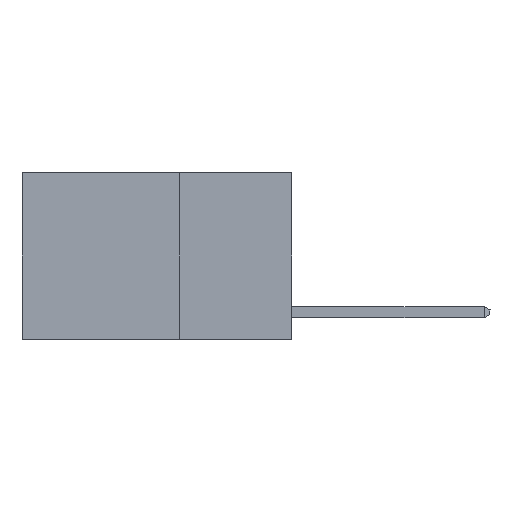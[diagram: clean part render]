
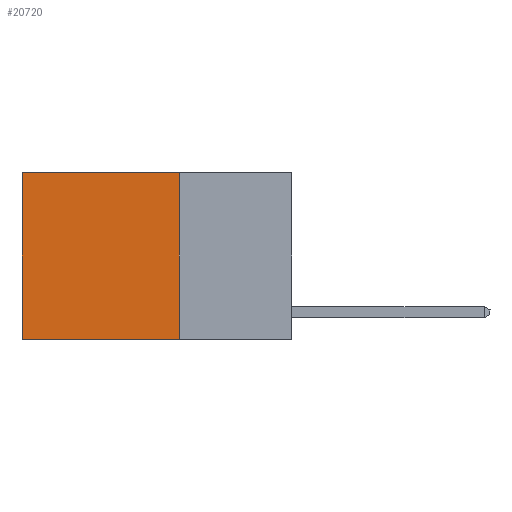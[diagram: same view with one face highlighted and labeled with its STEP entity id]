
A CAD part, left-side view. The second image highlights one B-rep face of the part: STEP entity #20720.
In plain terms, the highlighted planar face has unit normal (-1, 0, 0).
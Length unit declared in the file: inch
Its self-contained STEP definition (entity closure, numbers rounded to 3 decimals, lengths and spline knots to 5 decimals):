
#1170 = DIRECTION ( 'NONE',  ( 0., 0., -1. ) ) ;
#1508 = EDGE_CURVE ( 'NONE', #13375, #12511, #23772, .T. ) ;
#3871 = VECTOR ( 'NONE', #18918, 39.37008 ) ;
#3979 = VECTOR ( 'NONE', #27018, 39.37008 ) ;
#5860 = VECTOR ( 'NONE', #15550, 39.37008 ) ;
#6745 = AXIS2_PLACEMENT_3D ( 'NONE', #12817, #28065, #15003 ) ;
#6861 = CARTESIAN_POINT ( 'NONE',  ( 0.2625, 0.25, 0. ) ) ;
#7076 = CARTESIAN_POINT ( 'NONE',  ( 0.2625, 0.25, 0. ) ) ;
#10274 = ORIENTED_EDGE ( 'NONE', *, *, #1508, .T. ) ;
#11385 = EDGE_CURVE ( 'NONE', #13403, #13347, #15575, .T. ) ;
#12511 = VERTEX_POINT ( 'NONE', #22187 ) ;
#12817 = CARTESIAN_POINT ( 'NONE',  ( 0.2625, 0.25, 0. ) ) ;
#13039 = LINE ( 'NONE', #6861, #5860 ) ;
#13347 = VERTEX_POINT ( 'NONE', #24905 ) ;
#13375 = VERTEX_POINT ( 'NONE', #15666 ) ;
#13403 = VERTEX_POINT ( 'NONE', #7076 ) ;
#13899 = EDGE_CURVE ( 'NONE', #13403, #13375, #13039, .T. ) ;
#14240 = CARTESIAN_POINT ( 'NONE',  ( 0.2625, 0.6, 0. ) ) ;
#15003 = DIRECTION ( 'NONE',  ( 0., 0., -1. ) ) ;
#15550 = DIRECTION ( 'NONE',  ( 0., 1., 0. ) ) ;
#15575 = LINE ( 'NONE', #24815, #3979 ) ;
#15666 = CARTESIAN_POINT ( 'NONE',  ( 0.2625, 0.6, 0. ) ) ;
#18528 = ORIENTED_EDGE ( 'NONE', *, *, #13899, .T. ) ;
#18918 = DIRECTION ( 'NONE',  ( 0., 1., 0. ) ) ;
#19268 = EDGE_CURVE ( 'NONE', #13347, #12511, #27068, .T. ) ;
#20033 = VECTOR ( 'NONE', #1170, 39.37008 ) ;
#20720 = ADVANCED_FACE ( 'NONE', ( #22588 ), #21493, .F. ) ;
#21493 = PLANE ( 'NONE',  #6745 ) ;
#22187 = CARTESIAN_POINT ( 'NONE',  ( 0.2625, 0.6, -0.37 ) ) ;
#22588 = FACE_OUTER_BOUND ( 'NONE', #26997, .T. ) ;
#23768 = CARTESIAN_POINT ( 'NONE',  ( 0.2625, 0.25, -0.37 ) ) ;
#23772 = LINE ( 'NONE', #14240, #20033 ) ;
#24815 = CARTESIAN_POINT ( 'NONE',  ( 0.2625, 0.25, 0. ) ) ;
#24905 = CARTESIAN_POINT ( 'NONE',  ( 0.2625, 0.25, -0.37 ) ) ;
#26102 = ORIENTED_EDGE ( 'NONE', *, *, #19268, .F. ) ;
#26997 = EDGE_LOOP ( 'NONE', ( #10274, #26102, #28010, #18528 ) ) ;
#27018 = DIRECTION ( 'NONE',  ( 0., 0., -1. ) ) ;
#27068 = LINE ( 'NONE', #23768, #3871 ) ;
#28010 = ORIENTED_EDGE ( 'NONE', *, *, #11385, .F. ) ;
#28065 = DIRECTION ( 'NONE',  ( 1., 0., 0. ) ) ;
